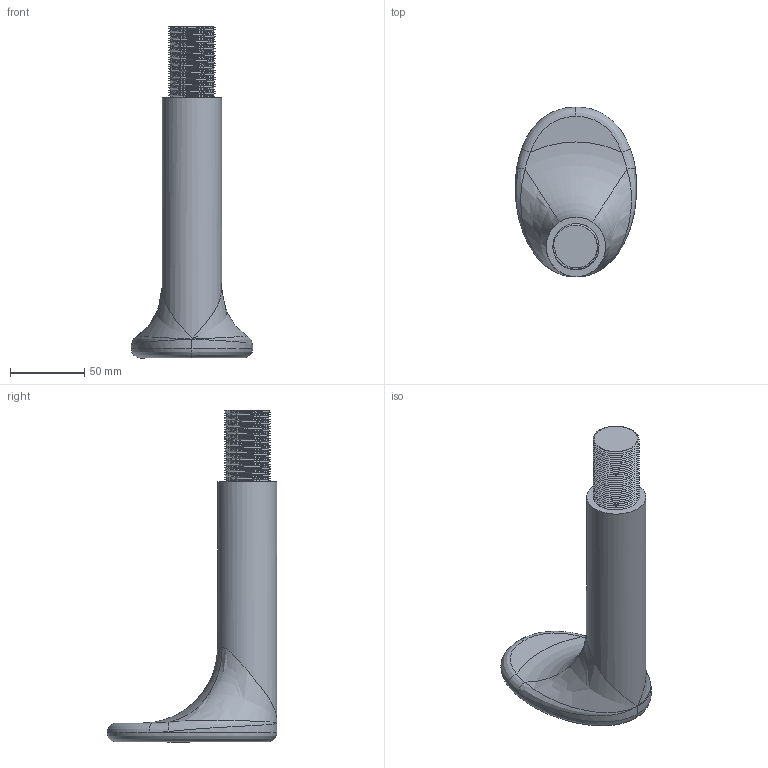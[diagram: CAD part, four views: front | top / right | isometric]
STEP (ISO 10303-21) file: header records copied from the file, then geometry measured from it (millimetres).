
FILE_DESCRIPTION (( 'STEP AP214' ), '1' );
FILE_NAME ('Threaded Stock.STEP', '2014-02-09T11:56:10', ( 'elpi' ), ( '' ), 'SwSTEP 2.0', 'SolidWorks 2013', '' );
FILE_SCHEMA (( 'AUTOMOTIVE_DESIGN' ));
Length unit declared in the file: inch
Products named in the file (1): Threaded Stock
Bounding box: 81.76 x 114.3 x 223.25 mm (x, y, z)
Volume: 284811.1 mm3; surface area: 59087.3 mm2
Topology: 1 solids, 1 shells, 102 faces, 277 edges, 175 vertices
Faces by surface type: cylinder 64, bspline 32, plane 5, torus 1
Full cylindrical faces by diameter (mm): 25.4 x1, 40 x1
Entity records: 24350 total; most frequent: CARTESIAN_POINT 21341, ORIENTED_EDGE 540, EDGE_CURVE 270, DIRECTION 236, VERTEX_POINT 174, EDGE_LOOP 106, FACE_OUTER_BOUND 104, ADVANCED_FACE 102
